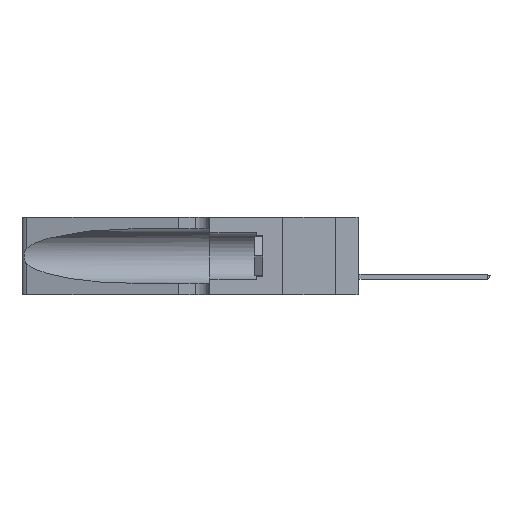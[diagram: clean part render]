
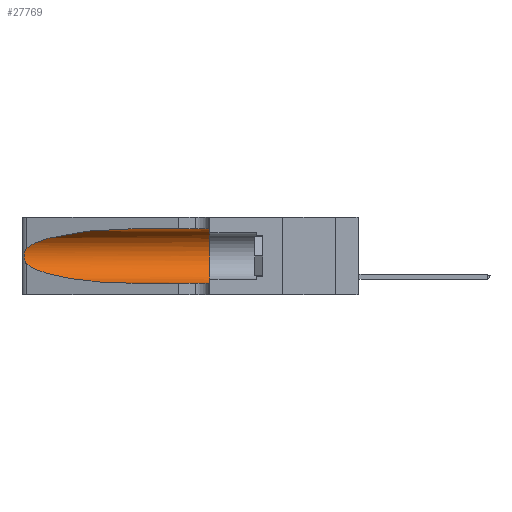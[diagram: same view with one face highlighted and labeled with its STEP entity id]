
A CAD part, left-side view. The second image highlights one B-rep face of the part: STEP entity #27769.
In plain terms, the highlighted cylindrical face has radius 3.308 mm (diameter 6.617 mm), a partial arc.
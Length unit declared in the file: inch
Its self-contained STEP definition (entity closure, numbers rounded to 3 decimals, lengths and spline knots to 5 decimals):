
#155 =( BOUNDED_CURVE ( )  B_SPLINE_CURVE ( 3, ( #28802, #9800, #34958, #16262 ),
 .UNSPECIFIED., .F., .F. ) 
 B_SPLINE_CURVE_WITH_KNOTS ( ( 4, 4 ),
 ( 3.44316, 4.71239 ),
 .UNSPECIFIED. ) 
 CURVE ( )  GEOMETRIC_REPRESENTATION_ITEM ( )  RATIONAL_B_SPLINE_CURVE ( ( 1., 0.87, 0.87, 1. ) ) 
 REPRESENTATION_ITEM ( '' )  );
#723 = CARTESIAN_POINT ( 'NONE',  ( 0.1305, 0.72297, 0.31525 ) ) ;
#779 = CARTESIAN_POINT ( 'NONE',  ( 0.25789, 1.23486, 0.15765 ) ) ;
#1865 = LINE ( 'NONE', #1874, #37318 ) ;
#1874 = CARTESIAN_POINT ( 'NONE',  ( 0.1305, 1.61858, 0.05475 ) ) ;
#2157 = VERTEX_POINT ( 'NONE', #13679 ) ;
#2849 = CARTESIAN_POINT ( 'NONE',  ( 0.18966, 0.96281, 0.31525 ) ) ;
#5309 = ORIENTED_EDGE ( 'NONE', *, *, #40207, .F. ) ;
#5549 = AXIS2_PLACEMENT_3D ( 'NONE', #12831, #28984, #9855 ) ;
#6943 = CARTESIAN_POINT ( 'NONE',  ( 0.25487, 1.22718, 0.22369 ) ) ;
#7320 = DIRECTION ( 'NONE',  ( 0., 0., 1. ) ) ;
#8107 = CARTESIAN_POINT ( 'NONE',  ( 0.25787, 1.23484, 0.2124 ) ) ;
#9800 = CARTESIAN_POINT ( 'NONE',  ( 0.2373, 1.15595, 0.08982 ) ) ;
#9855 = DIRECTION ( 'NONE',  ( 0., 0., -1. ) ) ;
#10083 = B_SPLINE_CURVE_WITH_KNOTS ( 'NONE', 3,
 ( #6943, #40700, #31787, #8107, #31567, #22701, #39096, #39220, #33609, #22587, #779, #29347, #13309, #29479 ),
 .UNSPECIFIED., .F., .F.,
 ( 4, 2, 2, 2, 2, 2, 4 ),
 ( 0., 0.00027, 0.00053, 0.00107, 0.0016, 0.00187, 0.00214 ),
 .UNSPECIFIED. ) ;
#12831 = CARTESIAN_POINT ( 'NONE',  ( 0.1305, 1.61858, 0.185 ) ) ;
#13309 = CARTESIAN_POINT ( 'NONE',  ( 0.25555, 1.22993, 0.14849 ) ) ;
#13679 = CARTESIAN_POINT ( 'NONE',  ( 0.25487, 1.22718, 0.14631 ) ) ;
#14117 = DIRECTION ( 'NONE',  ( 0., -1., 0. ) ) ;
#14322 = VERTEX_POINT ( 'NONE', #28922 ) ;
#15011 = ORIENTED_EDGE ( 'NONE', *, *, #30375, .F. ) ;
#15356 = VERTEX_POINT ( 'NONE', #39831 ) ;
#16115 = CARTESIAN_POINT ( 'NONE',  ( 0.1305, 0.72297, 0.31525 ) ) ;
#16180 = LINE ( 'NONE', #38513, #28668 ) ;
#16262 = CARTESIAN_POINT ( 'NONE',  ( 0.1305, 0.72297, 0.05475 ) ) ;
#16428 = VERTEX_POINT ( 'NONE', #34813 ) ;
#17134 = EDGE_CURVE ( 'NONE', #16428, #14322, #1865, .T. ) ;
#17234 = AXIS2_PLACEMENT_3D ( 'NONE', #32620, #29804, #7320 ) ;
#17651 = EDGE_CURVE ( 'NONE', #2157, #16428, #155, .T. ) ;
#19744 = CYLINDRICAL_SURFACE ( 'NONE', #5549, 0.13025 ) ;
#20448 = CARTESIAN_POINT ( 'NONE',  ( 0.25487, 1.22718, 0.22369 ) ) ;
#20743 = EDGE_LOOP ( 'NONE', ( #31384, #21334, #27831, #37647, #15011, #5309 ) ) ;
#21334 = ORIENTED_EDGE ( 'NONE', *, *, #26224, .T. ) ;
#22133 = CARTESIAN_POINT ( 'NONE',  ( 0.25487, 1.22718, 0.22369 ) ) ;
#22587 = CARTESIAN_POINT ( 'NONE',  ( 0.25856, 1.23593, 0.16098 ) ) ;
#22701 = CARTESIAN_POINT ( 'NONE',  ( 0.26018, 1.23835, 0.19895 ) ) ;
#26224 = EDGE_CURVE ( 'NONE', #39587, #2157, #10083, .T. ) ;
#26542 = CIRCLE ( 'NONE', #17234, 0.13025 ) ;
#27769 = ADVANCED_FACE ( 'NONE', ( #37218 ), #19744, .F. ) ;
#27831 = ORIENTED_EDGE ( 'NONE', *, *, #17651, .T. ) ;
#28668 = VECTOR ( 'NONE', #14117, 39.37008 ) ;
#28802 = CARTESIAN_POINT ( 'NONE',  ( 0.25487, 1.22718, 0.14631 ) ) ;
#28922 = CARTESIAN_POINT ( 'NONE',  ( 0.1305, 0.35, 0.05475 ) ) ;
#28984 = DIRECTION ( 'NONE',  ( 0., -1., 0. ) ) ;
#29347 = CARTESIAN_POINT ( 'NONE',  ( 0.25639, 1.23186, 0.15144 ) ) ;
#29479 = CARTESIAN_POINT ( 'NONE',  ( 0.25487, 1.22718, 0.14631 ) ) ;
#29546 = VERTEX_POINT ( 'NONE', #723 ) ;
#29804 = DIRECTION ( 'NONE',  ( 0., 1., 0. ) ) ;
#30375 = EDGE_CURVE ( 'NONE', #15356, #14322, #26542, .T. ) ;
#31192 = DIRECTION ( 'NONE',  ( 0., -1., 0. ) ) ;
#31384 = ORIENTED_EDGE ( 'NONE', *, *, #31468, .T. ) ;
#31468 = EDGE_CURVE ( 'NONE', #29546, #39587, #39750, .T. ) ;
#31567 = CARTESIAN_POINT ( 'NONE',  ( 0.25854, 1.2359, 0.20912 ) ) ;
#31787 = CARTESIAN_POINT ( 'NONE',  ( 0.25639, 1.23184, 0.21858 ) ) ;
#32620 = CARTESIAN_POINT ( 'NONE',  ( 0.1305, 0.35, 0.185 ) ) ;
#33609 = CARTESIAN_POINT ( 'NONE',  ( 0.26017, 1.23833, 0.17102 ) ) ;
#34678 = CARTESIAN_POINT ( 'NONE',  ( 0.2373, 1.15595, 0.28018 ) ) ;
#34813 = CARTESIAN_POINT ( 'NONE',  ( 0.1305, 0.72297, 0.05475 ) ) ;
#34958 = CARTESIAN_POINT ( 'NONE',  ( 0.18966, 0.96281, 0.05475 ) ) ;
#37218 = FACE_OUTER_BOUND ( 'NONE', #20743, .T. ) ;
#37318 = VECTOR ( 'NONE', #31192, 39.37008 ) ;
#37647 = ORIENTED_EDGE ( 'NONE', *, *, #17134, .T. ) ;
#38513 = CARTESIAN_POINT ( 'NONE',  ( 0.1305, 1.61858, 0.31525 ) ) ;
#39096 = CARTESIAN_POINT ( 'NONE',  ( 0.26075, 1.23896, 0.19203 ) ) ;
#39220 = CARTESIAN_POINT ( 'NONE',  ( 0.26075, 1.23896, 0.178 ) ) ;
#39587 = VERTEX_POINT ( 'NONE', #20448 ) ;
#39750 =( BOUNDED_CURVE ( )  B_SPLINE_CURVE ( 3, ( #16115, #2849, #34678, #22133 ),
 .UNSPECIFIED., .F., .T. ) 
 B_SPLINE_CURVE_WITH_KNOTS ( ( 4, 4 ),
 ( 1.5708, 2.84003 ),
 .UNSPECIFIED. ) 
 CURVE ( )  GEOMETRIC_REPRESENTATION_ITEM ( )  RATIONAL_B_SPLINE_CURVE ( ( 1., 0.87, 0.87, 1. ) ) 
 REPRESENTATION_ITEM ( '' )  );
#39831 = CARTESIAN_POINT ( 'NONE',  ( 0.1305, 0.35, 0.31525 ) ) ;
#40207 = EDGE_CURVE ( 'NONE', #29546, #15356, #16180, .T. ) ;
#40700 = CARTESIAN_POINT ( 'NONE',  ( 0.25555, 1.22994, 0.2215 ) ) ;
